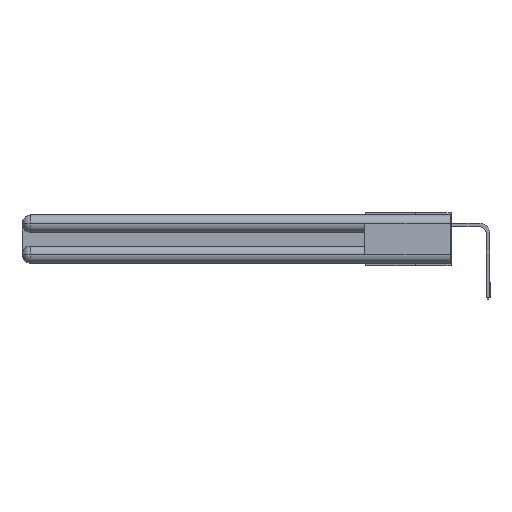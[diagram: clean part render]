
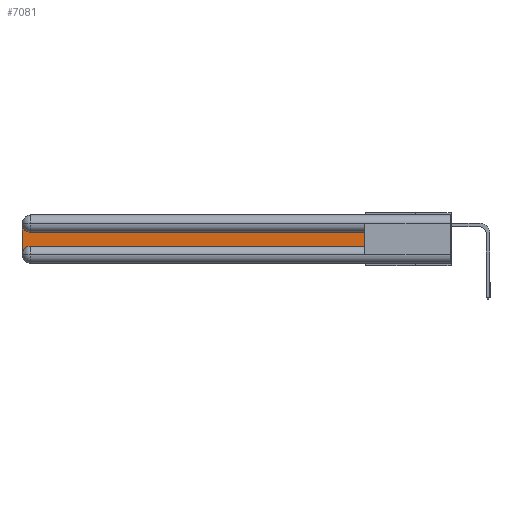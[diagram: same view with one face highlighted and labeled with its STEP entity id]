
A CAD part, left-side view. The second image highlights one B-rep face of the part: STEP entity #7081.
In plain terms, the highlighted planar face has unit normal (-1, 0, 0).
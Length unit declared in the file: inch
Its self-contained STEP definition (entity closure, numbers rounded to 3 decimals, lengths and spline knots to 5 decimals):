
#46 = VERTEX_POINT ( 'NONE', #1975 ) ;
#851 = EDGE_CURVE ( 'NONE', #16647, #9320, #19431, .T. ) ;
#1035 = DIRECTION ( 'NONE',  ( 0., -1., 0. ) ) ;
#1605 = AXIS2_PLACEMENT_3D ( 'NONE', #12483, #23524, #21331 ) ;
#1710 = DIRECTION ( 'NONE',  ( 0., 0., -1. ) ) ;
#1939 = VECTOR ( 'NONE', #1710, 39.37008 ) ;
#1975 = CARTESIAN_POINT ( 'NONE',  ( 0.075, 0.6, -0.1225 ) ) ;
#2119 = EDGE_LOOP ( 'NONE', ( #19496, #18671, #9147, #20633, #12673, #5166 ) ) ;
#2785 = AXIS2_PLACEMENT_3D ( 'NONE', #24166, #26286, #22057 ) ;
#2960 = DIRECTION ( 'NONE',  ( 1., 0., 0. ) ) ;
#3337 = VERTEX_POINT ( 'NONE', #27588 ) ;
#3434 = VERTEX_POINT ( 'NONE', #15523 ) ;
#4055 = CIRCLE ( 'NONE', #1605, 0.06 ) ;
#5166 = ORIENTED_EDGE ( 'NONE', *, *, #13176, .T. ) ;
#5871 = EDGE_CURVE ( 'NONE', #21901, #3337, #16976, .T. ) ;
#6003 = DIRECTION ( 'NONE',  ( 0., 0., 1. ) ) ;
#6193 = LINE ( 'NONE', #21005, #14115 ) ;
#7081 = ADVANCED_FACE ( 'NONE', ( #19641 ), #17405, .F. ) ;
#7338 = EDGE_CURVE ( 'NONE', #3434, #16647, #18645, .T. ) ;
#7559 = AXIS2_PLACEMENT_3D ( 'NONE', #18584, #2960, #27448 ) ;
#7681 = CARTESIAN_POINT ( 'NONE',  ( 0.075, 0.6, -0.2175 ) ) ;
#9147 = ORIENTED_EDGE ( 'NONE', *, *, #851, .T. ) ;
#9320 = VERTEX_POINT ( 'NONE', #26829 ) ;
#12483 = CARTESIAN_POINT ( 'NONE',  ( 0.075, 2.94, -0.2775 ) ) ;
#12601 = DIRECTION ( 'NONE',  ( 0., 1., 0. ) ) ;
#12673 = ORIENTED_EDGE ( 'NONE', *, *, #5871, .T. ) ;
#13176 = EDGE_CURVE ( 'NONE', #3337, #46, #16992, .T. ) ;
#14115 = VECTOR ( 'NONE', #12601, 39.37008 ) ;
#15523 = CARTESIAN_POINT ( 'NONE',  ( 0.075, 2.94, -0.1225 ) ) ;
#15572 = VECTOR ( 'NONE', #6003, 39.37008 ) ;
#16647 = VERTEX_POINT ( 'NONE', #28223 ) ;
#16969 = CARTESIAN_POINT ( 'NONE',  ( 0.075, 3., -0.2175 ) ) ;
#16976 = LINE ( 'NONE', #7681, #22739 ) ;
#16992 = LINE ( 'NONE', #28225, #15572 ) ;
#17405 = PLANE ( 'NONE',  #2785 ) ;
#18584 = CARTESIAN_POINT ( 'NONE',  ( 0.075, 2.94, -0.0625 ) ) ;
#18645 = CIRCLE ( 'NONE', #7559, 0.06 ) ;
#18671 = ORIENTED_EDGE ( 'NONE', *, *, #7338, .T. ) ;
#19431 = LINE ( 'NONE', #16969, #1939 ) ;
#19496 = ORIENTED_EDGE ( 'NONE', *, *, #23648, .T. ) ;
#19641 = FACE_OUTER_BOUND ( 'NONE', #2119, .T. ) ;
#20633 = ORIENTED_EDGE ( 'NONE', *, *, #26815, .T. ) ;
#21005 = CARTESIAN_POINT ( 'NONE',  ( 0.075, 0.6, -0.1225 ) ) ;
#21331 = DIRECTION ( 'NONE',  ( 0., 0., -1. ) ) ;
#21901 = VERTEX_POINT ( 'NONE', #23978 ) ;
#22057 = DIRECTION ( 'NONE',  ( 0., 0., -1. ) ) ;
#22739 = VECTOR ( 'NONE', #1035, 39.37008 ) ;
#23524 = DIRECTION ( 'NONE',  ( 1., 0., 0. ) ) ;
#23648 = EDGE_CURVE ( 'NONE', #46, #3434, #6193, .T. ) ;
#23978 = CARTESIAN_POINT ( 'NONE',  ( 0.075, 2.94, -0.2175 ) ) ;
#24166 = CARTESIAN_POINT ( 'NONE',  ( 0.075, 3., -0.1225 ) ) ;
#26286 = DIRECTION ( 'NONE',  ( 1., 0., 0. ) ) ;
#26815 = EDGE_CURVE ( 'NONE', #9320, #21901, #4055, .T. ) ;
#26829 = CARTESIAN_POINT ( 'NONE',  ( 0.075, 3., -0.2775 ) ) ;
#27448 = DIRECTION ( 'NONE',  ( 0., 0., -1. ) ) ;
#27588 = CARTESIAN_POINT ( 'NONE',  ( 0.075, 0.6, -0.2175 ) ) ;
#28223 = CARTESIAN_POINT ( 'NONE',  ( 0.075, 3., -0.0625 ) ) ;
#28225 = CARTESIAN_POINT ( 'NONE',  ( 0.075, 0.6, -0.2175 ) ) ;
